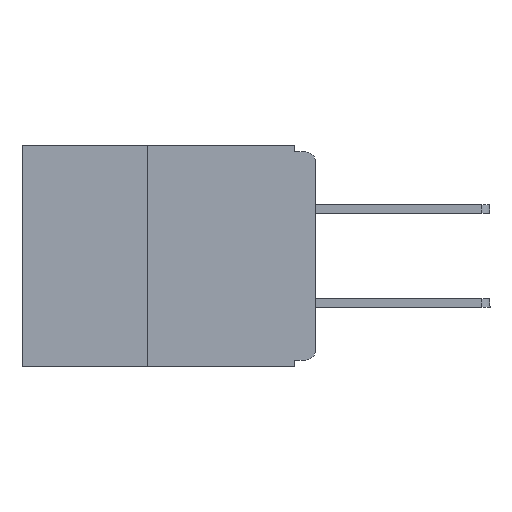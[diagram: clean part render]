
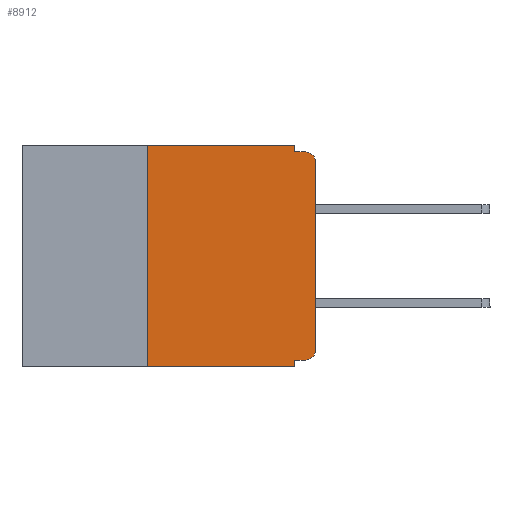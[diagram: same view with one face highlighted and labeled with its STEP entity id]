
A CAD part, left-side view. The second image highlights one B-rep face of the part: STEP entity #8912.
In plain terms, the highlighted planar face has unit normal (-1, 0, 0).
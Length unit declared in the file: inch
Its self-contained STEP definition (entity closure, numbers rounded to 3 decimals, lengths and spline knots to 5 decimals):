
#97 = VECTOR ( 'NONE', #8996, 39.37008 ) ;
#119 = CARTESIAN_POINT ( 'NONE',  ( 0., 0.015, -0.01 ) ) ;
#136 = VERTEX_POINT ( 'NONE', #6131 ) ;
#304 = VECTOR ( 'NONE', #9450, 39.37008 ) ;
#382 = EDGE_CURVE ( 'NONE', #11648, #1756, #4406, .T. ) ;
#438 = EDGE_CURVE ( 'NONE', #136, #11154, #6379, .T. ) ;
#554 = CARTESIAN_POINT ( 'NONE',  ( 0., 0.437, -0.33 ) ) ;
#662 = DIRECTION ( 'NONE',  ( 0., 0., -1. ) ) ;
#767 = VECTOR ( 'NONE', #3203, 39.37008 ) ;
#1051 = CARTESIAN_POINT ( 'NONE',  ( 0., 0.25, 0. ) ) ;
#1411 = CARTESIAN_POINT ( 'NONE',  ( 0., 0., -0.01 ) ) ;
#1756 = VERTEX_POINT ( 'NONE', #119 ) ;
#2007 = DIRECTION ( 'NONE',  ( 1., 0., 0. ) ) ;
#2012 = ORIENTED_EDGE ( 'NONE', *, *, #3550, .T. ) ;
#2068 = EDGE_CURVE ( 'NONE', #6799, #10090, #12156, .T. ) ;
#2122 = LINE ( 'NONE', #3401, #2510 ) ;
#2171 = ORIENTED_EDGE ( 'NONE', *, *, #10320, .T. ) ;
#2269 = ORIENTED_EDGE ( 'NONE', *, *, #382, .F. ) ;
#2385 = ORIENTED_EDGE ( 'NONE', *, *, #2717, .F. ) ;
#2502 = ORIENTED_EDGE ( 'NONE', *, *, #5344, .F. ) ;
#2510 = VECTOR ( 'NONE', #4333, 39.37008 ) ;
#2717 = EDGE_CURVE ( 'NONE', #6387, #11648, #2122, .T. ) ;
#2778 = ORIENTED_EDGE ( 'NONE', *, *, #438, .F. ) ;
#2819 = CARTESIAN_POINT ( 'NONE',  ( 0., 0., 0. ) ) ;
#2838 = VERTEX_POINT ( 'NONE', #8026 ) ;
#2881 = ORIENTED_EDGE ( 'NONE', *, *, #7193, .T. ) ;
#3203 = DIRECTION ( 'NONE',  ( 0., -1., 0. ) ) ;
#3231 = LINE ( 'NONE', #2819, #97 ) ;
#3273 = EDGE_CURVE ( 'NONE', #2838, #6799, #12466, .T. ) ;
#3401 = CARTESIAN_POINT ( 'NONE',  ( 0., 0.031, 0. ) ) ;
#3540 = ORIENTED_EDGE ( 'NONE', *, *, #2068, .F. ) ;
#3550 = EDGE_CURVE ( 'NONE', #5039, #11730, #3231, .T. ) ;
#3641 = ORIENTED_EDGE ( 'NONE', *, *, #3273, .F. ) ;
#3804 = VECTOR ( 'NONE', #9402, 39.37008 ) ;
#3865 = LINE ( 'NONE', #554, #11868 ) ;
#3972 = ORIENTED_EDGE ( 'NONE', *, *, #12290, .T. ) ;
#4130 = AXIS2_PLACEMENT_3D ( 'NONE', #12175, #5767, #13223 ) ;
#4333 = DIRECTION ( 'NONE',  ( 0., 0., -1. ) ) ;
#4406 = LINE ( 'NONE', #1411, #12691 ) ;
#4466 = CARTESIAN_POINT ( 'NONE',  ( 0., 0.031, -0.33 ) ) ;
#4839 = CIRCLE ( 'NONE', #11941, 0.015 ) ;
#5039 = VERTEX_POINT ( 'NONE', #13989 ) ;
#5344 = EDGE_CURVE ( 'NONE', #11154, #6387, #12244, .T. ) ;
#5767 = DIRECTION ( 'NONE',  ( -1., 0., 0. ) ) ;
#6112 = DIRECTION ( 'NONE',  ( 0., -1., 0. ) ) ;
#6131 = CARTESIAN_POINT ( 'NONE',  ( 0., 0.25, -0.33 ) ) ;
#6244 = CARTESIAN_POINT ( 'NONE',  ( 0., 0.25, -0.33 ) ) ;
#6379 = LINE ( 'NONE', #6244, #12036 ) ;
#6387 = VERTEX_POINT ( 'NONE', #11033 ) ;
#6587 = CARTESIAN_POINT ( 'NONE',  ( 0., 0.437, 0. ) ) ;
#6799 = VERTEX_POINT ( 'NONE', #14189 ) ;
#7067 = CIRCLE ( 'NONE', #4130, 0.015 ) ;
#7193 = EDGE_CURVE ( 'NONE', #136, #10090, #3865, .T. ) ;
#7583 = DIRECTION ( 'NONE',  ( -1., 0., 0. ) ) ;
#7966 = DIRECTION ( 'NONE',  ( 0., -1., 0. ) ) ;
#8026 = CARTESIAN_POINT ( 'NONE',  ( 0., 0.015, -0.32 ) ) ;
#8815 = PLANE ( 'NONE',  #11838 ) ;
#8912 = ADVANCED_FACE ( 'NONE', ( #12141 ), #8815, .F. ) ;
#8996 = DIRECTION ( 'NONE',  ( 0., 0., 1. ) ) ;
#9402 = DIRECTION ( 'NONE',  ( 0., 1., 0. ) ) ;
#9414 = CARTESIAN_POINT ( 'NONE',  ( 0., 0.031, -0.33 ) ) ;
#9450 = DIRECTION ( 'NONE',  ( 0., 0., -1. ) ) ;
#9603 = CARTESIAN_POINT ( 'NONE',  ( 0., 0., -0.32 ) ) ;
#9691 = EDGE_LOOP ( 'NONE', ( #2012, #2171, #2269, #2385, #2502, #2778, #2881, #3540, #3641, #3972 ) ) ;
#9872 = DIRECTION ( 'NONE',  ( 0., 0., -1. ) ) ;
#9981 = DIRECTION ( 'NONE',  ( 0., 0., 1. ) ) ;
#10090 = VERTEX_POINT ( 'NONE', #4466 ) ;
#10320 = EDGE_CURVE ( 'NONE', #11730, #1756, #4839, .T. ) ;
#10993 = CARTESIAN_POINT ( 'NONE',  ( 0., 0., -0.025 ) ) ;
#11033 = CARTESIAN_POINT ( 'NONE',  ( 0., 0.031, 0. ) ) ;
#11154 = VERTEX_POINT ( 'NONE', #1051 ) ;
#11648 = VERTEX_POINT ( 'NONE', #13861 ) ;
#11730 = VERTEX_POINT ( 'NONE', #10993 ) ;
#11838 = AXIS2_PLACEMENT_3D ( 'NONE', #12995, #2007, #9872 ) ;
#11868 = VECTOR ( 'NONE', #6112, 39.37008 ) ;
#11941 = AXIS2_PLACEMENT_3D ( 'NONE', #13805, #7583, #662 ) ;
#12036 = VECTOR ( 'NONE', #9981, 39.37008 ) ;
#12141 = FACE_OUTER_BOUND ( 'NONE', #9691, .T. ) ;
#12156 = LINE ( 'NONE', #9414, #304 ) ;
#12175 = CARTESIAN_POINT ( 'NONE',  ( 0., 0.015, -0.305 ) ) ;
#12244 = LINE ( 'NONE', #6587, #767 ) ;
#12290 = EDGE_CURVE ( 'NONE', #2838, #5039, #7067, .T. ) ;
#12466 = LINE ( 'NONE', #9603, #3804 ) ;
#12691 = VECTOR ( 'NONE', #7966, 39.37008 ) ;
#12995 = CARTESIAN_POINT ( 'NONE',  ( 0., 0.437, 0. ) ) ;
#13223 = DIRECTION ( 'NONE',  ( 0., 0., -1. ) ) ;
#13805 = CARTESIAN_POINT ( 'NONE',  ( 0., 0.015, -0.025 ) ) ;
#13861 = CARTESIAN_POINT ( 'NONE',  ( 0., 0.031, -0.01 ) ) ;
#13989 = CARTESIAN_POINT ( 'NONE',  ( 0., 0., -0.305 ) ) ;
#14189 = CARTESIAN_POINT ( 'NONE',  ( 0., 0.031, -0.32 ) ) ;
